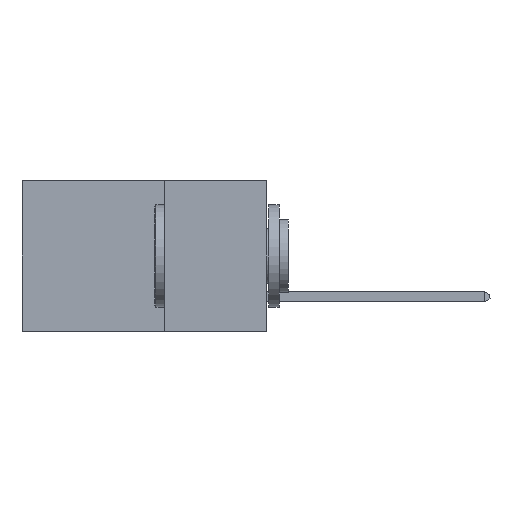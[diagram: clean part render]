
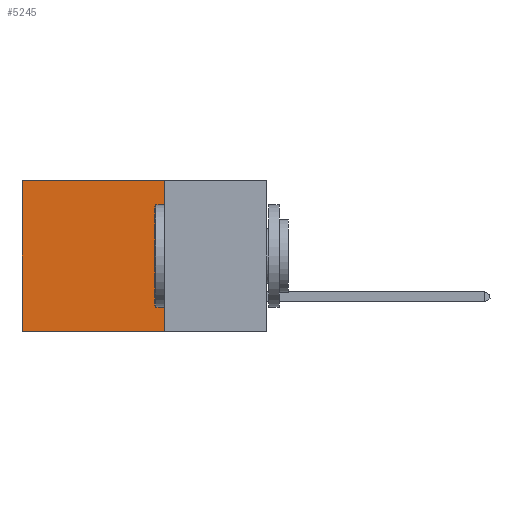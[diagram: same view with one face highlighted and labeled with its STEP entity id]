
A CAD part, left-side view. The second image highlights one B-rep face of the part: STEP entity #5245.
In plain terms, the highlighted planar face has unit normal (-1, 0, 0).
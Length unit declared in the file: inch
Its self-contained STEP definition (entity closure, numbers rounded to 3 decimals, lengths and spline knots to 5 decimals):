
#849 = EDGE_CURVE ( 'NONE', #3027, #1427, #10901, .T. ) ;
#1049 = VECTOR ( 'NONE', #5428, 39.37008 ) ;
#1378 = EDGE_CURVE ( 'NONE', #5053, #1427, #10778, .T. ) ;
#1427 = VERTEX_POINT ( 'NONE', #9021 ) ;
#2716 = CARTESIAN_POINT ( 'NONE',  ( 0.2875, 0.25, 0. ) ) ;
#3027 = VERTEX_POINT ( 'NONE', #11090 ) ;
#3709 = DIRECTION ( 'NONE',  ( 0., 1., 0. ) ) ;
#3939 = EDGE_CURVE ( 'NONE', #7554, #3027, #8555, .T. ) ;
#4146 = CARTESIAN_POINT ( 'NONE',  ( 0.2875, 0.25, 0. ) ) ;
#4254 = CARTESIAN_POINT ( 'NONE',  ( 0.2875, 0.6, 0. ) ) ;
#4256 = ORIENTED_EDGE ( 'NONE', *, *, #1378, .T. ) ;
#4266 = ORIENTED_EDGE ( 'NONE', *, *, #849, .F. ) ;
#4418 = ORIENTED_EDGE ( 'NONE', *, *, #3939, .F. ) ;
#4429 = ORIENTED_EDGE ( 'NONE', *, *, #10542, .T. ) ;
#4459 = FACE_OUTER_BOUND ( 'NONE', #6745, .T. ) ;
#4861 = LINE ( 'NONE', #2716, #11131 ) ;
#5053 = VERTEX_POINT ( 'NONE', #4254 ) ;
#5245 = ADVANCED_FACE ( 'NONE', ( #4459 ), #11906, .F. ) ;
#5272 = CARTESIAN_POINT ( 'NONE',  ( 0.2875, 0.25, 0. ) ) ;
#5428 = DIRECTION ( 'NONE',  ( 0., 0., -1. ) ) ;
#5628 = DIRECTION ( 'NONE',  ( 0., 1., 0. ) ) ;
#6093 = VECTOR ( 'NONE', #6191, 39.37008 ) ;
#6191 = DIRECTION ( 'NONE',  ( 0., 0., -1. ) ) ;
#6745 = EDGE_LOOP ( 'NONE', ( #4256, #4266, #4418, #4429 ) ) ;
#6845 = CARTESIAN_POINT ( 'NONE',  ( 0.2875, 0.6, 0. ) ) ;
#7554 = VERTEX_POINT ( 'NONE', #4146 ) ;
#8118 = CARTESIAN_POINT ( 'NONE',  ( 0.2875, 0.25, -0.37 ) ) ;
#8555 = LINE ( 'NONE', #5272, #1049 ) ;
#9021 = CARTESIAN_POINT ( 'NONE',  ( 0.2875, 0.6, -0.37 ) ) ;
#9272 = AXIS2_PLACEMENT_3D ( 'NONE', #11898, #11860, #11851 ) ;
#10526 = VECTOR ( 'NONE', #5628, 39.37008 ) ;
#10542 = EDGE_CURVE ( 'NONE', #7554, #5053, #4861, .T. ) ;
#10778 = LINE ( 'NONE', #6845, #6093 ) ;
#10901 = LINE ( 'NONE', #8118, #10526 ) ;
#11090 = CARTESIAN_POINT ( 'NONE',  ( 0.2875, 0.25, -0.37 ) ) ;
#11131 = VECTOR ( 'NONE', #3709, 39.37008 ) ;
#11851 = DIRECTION ( 'NONE',  ( 0., 0., -1. ) ) ;
#11860 = DIRECTION ( 'NONE',  ( 1., 0., 0. ) ) ;
#11898 = CARTESIAN_POINT ( 'NONE',  ( 0.2875, 0.25, 0. ) ) ;
#11906 = PLANE ( 'NONE',  #9272 ) ;
